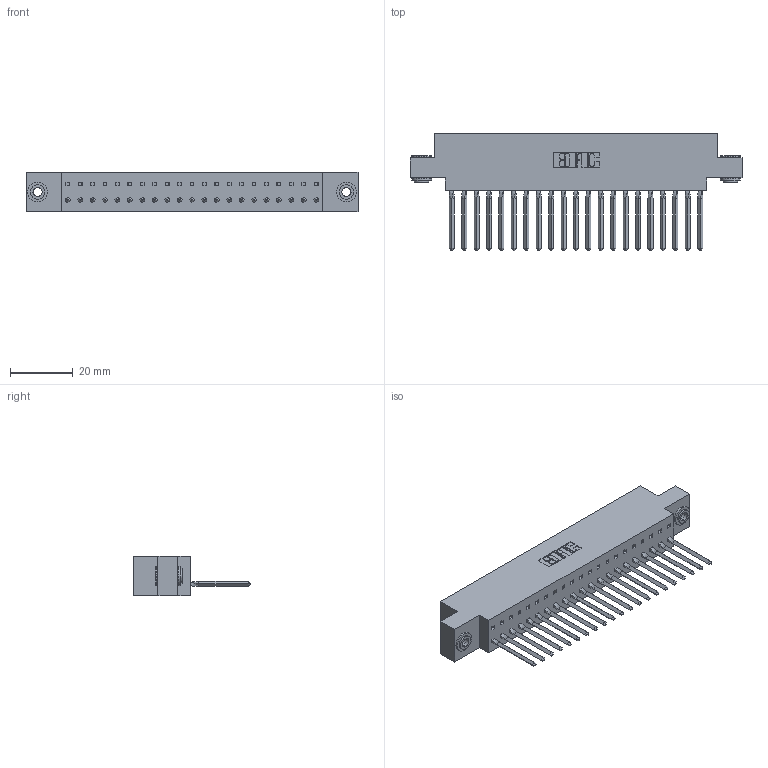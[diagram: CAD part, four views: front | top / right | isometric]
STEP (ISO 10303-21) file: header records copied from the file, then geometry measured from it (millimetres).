
FILE_DESCRIPTION (( 'STEP AP203' ), '1' );
FILE_NAME ('317-021-541-603.STEP', '2020-02-27T17:03:59', ( '' ), ( '' ), 'SwSTEP 2.0', 'SolidWorks 2016', '' );
FILE_SCHEMA (( 'CONFIG_CONTROL_DESIGN' ));
Length unit declared in the file: inch
Products named in the file (4): 345-250-002_345-250-002-102; 317 Part_.156 Dia - TH; 317-290-002_541; 317-021-541-603
Assembly tree (24 placements, depth 2):
  317-021-541-603
    317 Part_.156 Dia - TH
    317-290-002_541  x21
    345-250-002_345-250-002-102  x2
Bounding box: 105.92 x 37.34 x 12.7 mm (x, y, z)
Volume: 16550 mm3; surface area: 22900.8 mm2
Topology: 24 solids, 24 shells, 3332 faces, 9465 edges, 6152 vertices
Faces by surface type: plane 2672, cylinder 568, bspline 84, cone 8
Entity records: 34811 total; most frequent: CARTESIAN_POINT 6787, ORIENTED_EDGE 6054, DIRECTION 4999, EDGE_CURVE 3027, LINE 2639, VECTOR 2639, VERTEX_POINT 2008, AXIS2_PLACEMENT_3D 1180
